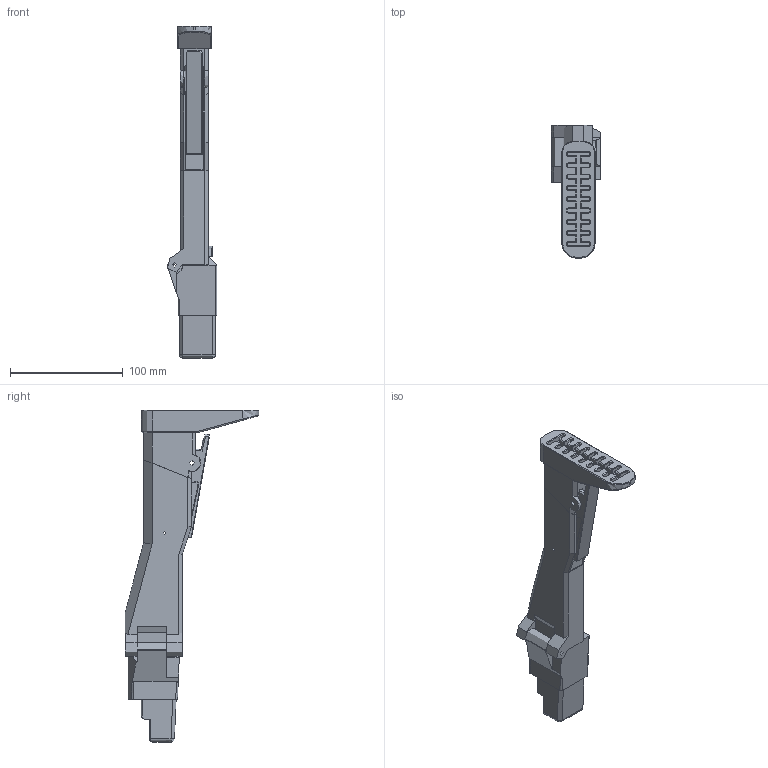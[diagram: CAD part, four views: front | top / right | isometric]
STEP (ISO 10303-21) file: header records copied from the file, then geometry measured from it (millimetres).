
FILE_DESCRIPTION(/* description */ (''),/* implementation_level */ '2;1');
FILE_NAME(/* name */ 'AKM FOLDING STOCK.stp',/* time_stamp */ '2021-03-20T21:59:26+01:00',/* author */ (''),/* organization */ (''),/* preprocessor_version */ 'ST-DEVELOPER v15.2',/* originating_system */ 'Autodesk Translator Framework v2.0.0.5431',/* authorisation */ '');
FILE_SCHEMA (('AUTOMOTIVE_DESIGN { 1 0 10303 214 3 1 1 }'));
Length unit declared in the file: centimetre
Products named in the file (1): abc
Bounding box: 43.88 x 118.38 x 294.51 mm (x, y, z)
Volume: 331447.7 mm3; surface area: 99872.1 mm2
Topology: 6 solids, 6 shells, 785 faces, 2037 edges, 1284 vertices
Faces by surface type: plane 485, cylinder 174, cone 82, bspline 24, torus 16, sphere 4
Full cylindrical faces by diameter (mm): 2.2 x2, 3 x2, 4 x5, 4.4 x4, 6.4 x1, 6.6 x1, 7 x1, 12.1 x1, 20.5 x1
Entity records: 24632 total; most frequent: CARTESIAN_POINT 5322, ORIENTED_EDGE 4018, DIRECTION 3968, EDGE_CURVE 2009, LINE 1454, VECTOR 1454, VERTEX_POINT 1278, AXIS2_PLACEMENT_3D 1257
